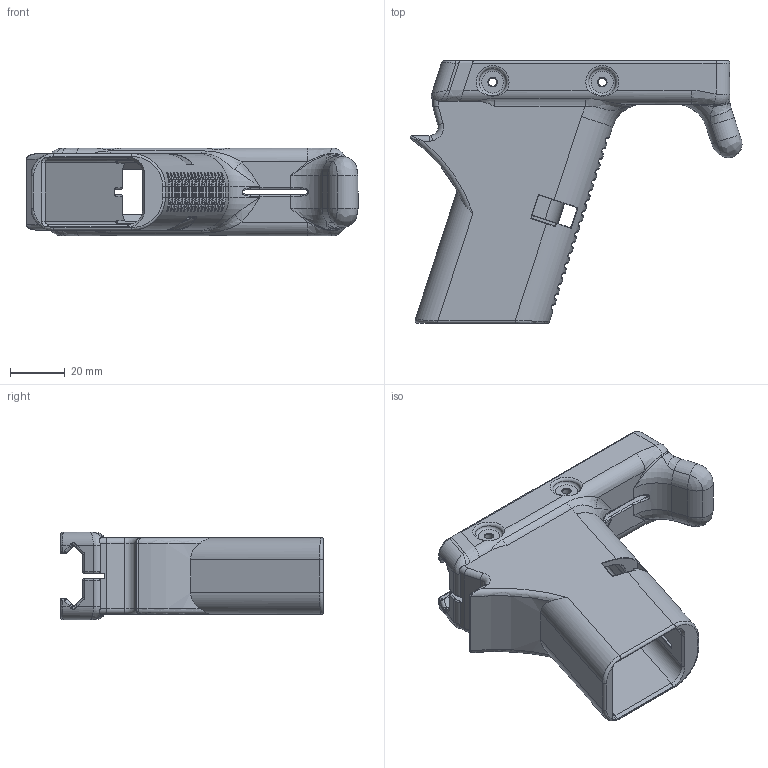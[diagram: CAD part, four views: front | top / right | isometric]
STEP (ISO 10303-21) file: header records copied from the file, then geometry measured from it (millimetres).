
FILE_DESCRIPTION(/* description */ (''),/* implementation_level */ '2;1');
FILE_NAME(/* name */ 'G17L PDW 2 Mag Holder.step',/* time_stamp */ '2021-05-20T09:27:54-06:00',/* author */ (''),/* organization */ (''),/* preprocessor_version */ 'ST-DEVELOPER v18.1',/* originating_system */ 'Autodesk Translation Framework v10.6.0.1341',/* authorisation */ '');
FILE_SCHEMA (('AUTOMOTIVE_DESIGN { 1 0 10303 214 3 1 1 }'));
Length unit declared in the file: millimetre
Products named in the file (1): G17L PDW 3
Bounding box: 121.12 x 95.85 x 32 mm (x, y, z)
Volume: 637.4 mm3; surface area: 35938.4 mm2
Topology: 1 solids, 2 shells, 772 faces, 1962 edges, 1151 vertices
Faces by surface type: bspline 274, cylinder 251, plane 173, torus 57, sphere 13, cone 4
Full cylindrical faces by diameter (mm): 3 x4
Entity records: 35524 total; most frequent: CARTESIAN_POINT 18082, ORIENTED_EDGE 3896, DIRECTION 3371, EDGE_CURVE 1932, AXIS2_PLACEMENT_3D 1348, VERTEX_POINT 1151, EDGE_LOOP 776, FACE_OUTER_BOUND 772
